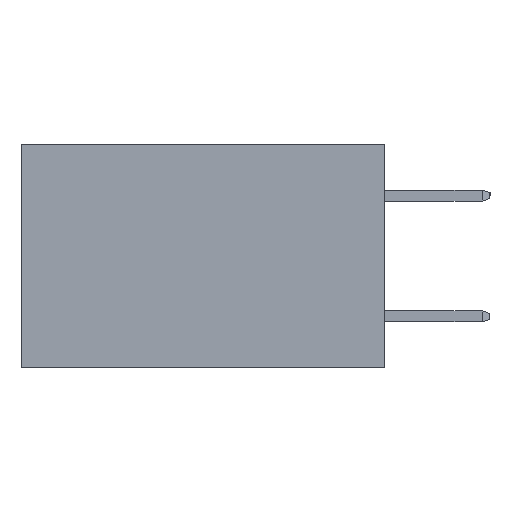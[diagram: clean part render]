
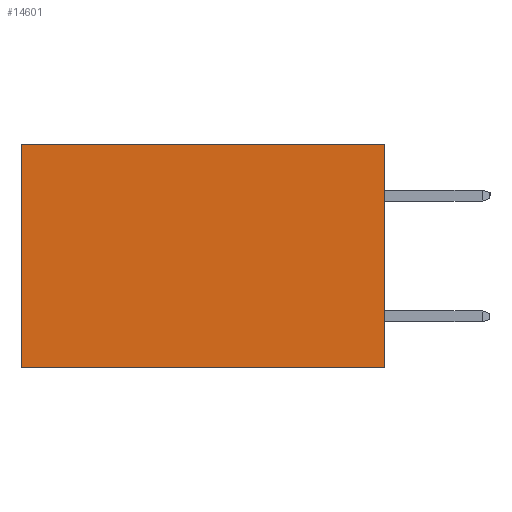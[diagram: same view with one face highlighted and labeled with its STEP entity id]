
A CAD part, left-side view. The second image highlights one B-rep face of the part: STEP entity #14601.
In plain terms, the highlighted planar face has unit normal (-1, 0, 0).
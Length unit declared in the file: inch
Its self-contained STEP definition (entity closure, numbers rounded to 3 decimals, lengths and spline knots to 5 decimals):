
#670 = DIRECTION ( 'NONE',  ( 0., 0., -1. ) ) ;
#1157 = AXIS2_PLACEMENT_3D ( 'NONE', #3031, #11463, #670 ) ;
#1230 = VECTOR ( 'NONE', #15475, 39.37008 ) ;
#3031 = CARTESIAN_POINT ( 'NONE',  ( 0.2615, 0., -0.37 ) ) ;
#3240 = VECTOR ( 'NONE', #4935, 39.37008 ) ;
#3587 = DIRECTION ( 'NONE',  ( 0., 1., 0. ) ) ;
#4126 = LINE ( 'NONE', #8133, #14610 ) ;
#4935 = DIRECTION ( 'NONE',  ( 0., 1., 0. ) ) ;
#5660 = EDGE_CURVE ( 'NONE', #11619, #14090, #19087, .T. ) ;
#6994 = CARTESIAN_POINT ( 'NONE',  ( 0.2615, 0., 0. ) ) ;
#7462 = LINE ( 'NONE', #15907, #18947 ) ;
#8133 = CARTESIAN_POINT ( 'NONE',  ( 0.2615, 0.6, -0.37 ) ) ;
#8777 = ORIENTED_EDGE ( 'NONE', *, *, #19409, .F. ) ;
#8980 = ORIENTED_EDGE ( 'NONE', *, *, #5660, .F. ) ;
#11463 = DIRECTION ( 'NONE',  ( 1., 0., 0. ) ) ;
#11619 = VERTEX_POINT ( 'NONE', #13606 ) ;
#12558 = DIRECTION ( 'NONE',  ( 0., 0., -1. ) ) ;
#13606 = CARTESIAN_POINT ( 'NONE',  ( 0.2615, 0., 0. ) ) ;
#14090 = VERTEX_POINT ( 'NONE', #21759 ) ;
#14601 = ADVANCED_FACE ( 'NONE', ( #15342 ), #23791, .F. ) ;
#14610 = VECTOR ( 'NONE', #12558, 39.37008 ) ;
#14905 = CARTESIAN_POINT ( 'NONE',  ( 0.2615, 0., -0.37 ) ) ;
#15342 = FACE_OUTER_BOUND ( 'NONE', #16208, .T. ) ;
#15475 = DIRECTION ( 'NONE',  ( 0., 0., -1. ) ) ;
#15907 = CARTESIAN_POINT ( 'NONE',  ( 0.2615, 0., -0.37 ) ) ;
#15925 = ORIENTED_EDGE ( 'NONE', *, *, #21561, .T. ) ;
#16208 = EDGE_LOOP ( 'NONE', ( #21006, #8777, #8980, #15925 ) ) ;
#16609 = CARTESIAN_POINT ( 'NONE',  ( 0.2615, 0.6, -0.37 ) ) ;
#18947 = VECTOR ( 'NONE', #3587, 39.37008 ) ;
#19087 = LINE ( 'NONE', #14905, #1230 ) ;
#19409 = EDGE_CURVE ( 'NONE', #14090, #25055, #7462, .T. ) ;
#20985 = EDGE_CURVE ( 'NONE', #23074, #25055, #4126, .T. ) ;
#21006 = ORIENTED_EDGE ( 'NONE', *, *, #20985, .T. ) ;
#21561 = EDGE_CURVE ( 'NONE', #11619, #23074, #25965, .T. ) ;
#21759 = CARTESIAN_POINT ( 'NONE',  ( 0.2615, 0., -0.37 ) ) ;
#23074 = VERTEX_POINT ( 'NONE', #23446 ) ;
#23446 = CARTESIAN_POINT ( 'NONE',  ( 0.2615, 0.6, 0. ) ) ;
#23791 = PLANE ( 'NONE',  #1157 ) ;
#25055 = VERTEX_POINT ( 'NONE', #16609 ) ;
#25965 = LINE ( 'NONE', #6994, #3240 ) ;
